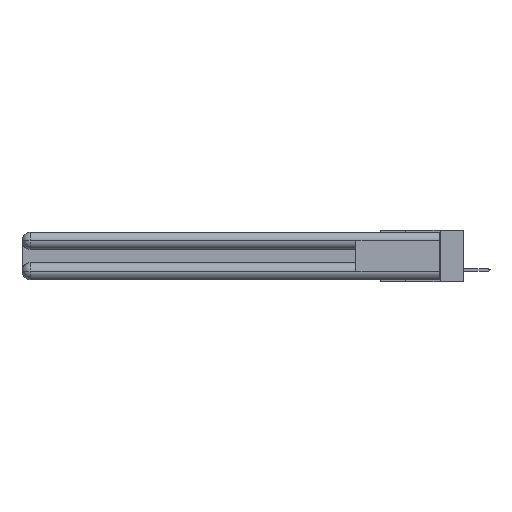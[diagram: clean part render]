
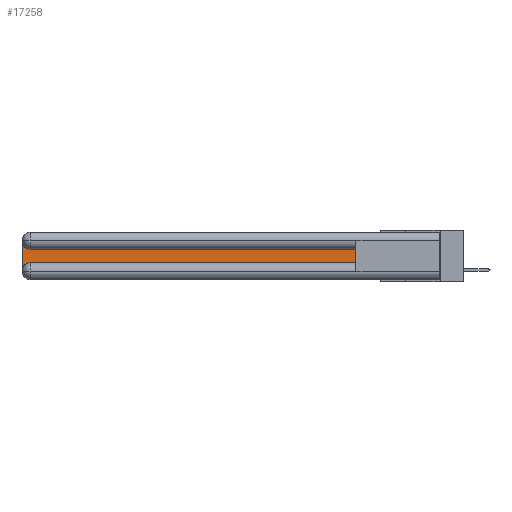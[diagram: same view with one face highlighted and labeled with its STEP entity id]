
A CAD part, left-side view. The second image highlights one B-rep face of the part: STEP entity #17258.
In plain terms, the highlighted planar face has unit normal (-1, 0, 0).
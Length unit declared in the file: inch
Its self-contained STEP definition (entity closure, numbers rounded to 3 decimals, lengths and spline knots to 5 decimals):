
#120 = DIRECTION ( 'NONE',  ( 0., 1., 0. ) ) ;
#713 = ORIENTED_EDGE ( 'NONE', *, *, #8002, .T. ) ;
#2307 = VECTOR ( 'NONE', #11723, 39.37008 ) ;
#2457 = PLANE ( 'NONE',  #19651 ) ;
#3687 = CARTESIAN_POINT ( 'NONE',  ( 0.075, 3., -0.2775 ) ) ;
#3909 = ORIENTED_EDGE ( 'NONE', *, *, #23828, .T. ) ;
#4156 = VERTEX_POINT ( 'NONE', #4724 ) ;
#4724 = CARTESIAN_POINT ( 'NONE',  ( 0.075, 3., -0.0625 ) ) ;
#6380 = LINE ( 'NONE', #19947, #2307 ) ;
#6751 = CARTESIAN_POINT ( 'NONE',  ( 0.075, 0.6, -0.1225 ) ) ;
#7042 = CARTESIAN_POINT ( 'NONE',  ( 0.075, 0.6, -0.2175 ) ) ;
#7141 = VECTOR ( 'NONE', #120, 39.37008 ) ;
#8002 = EDGE_CURVE ( 'NONE', #8964, #11441, #6380, .T. ) ;
#8964 = VERTEX_POINT ( 'NONE', #19576 ) ;
#9056 = DIRECTION ( 'NONE',  ( 0., 0., -1. ) ) ;
#9434 = LINE ( 'NONE', #7042, #18223 ) ;
#9610 = VECTOR ( 'NONE', #18591, 39.37008 ) ;
#9648 = ORIENTED_EDGE ( 'NONE', *, *, #23434, .T. ) ;
#10524 = CIRCLE ( 'NONE', #25186, 0.06 ) ;
#11144 = CIRCLE ( 'NONE', #14987, 0.06 ) ;
#11259 = VERTEX_POINT ( 'NONE', #6751 ) ;
#11441 = VERTEX_POINT ( 'NONE', #24611 ) ;
#11643 = ORIENTED_EDGE ( 'NONE', *, *, #21278, .T. ) ;
#11723 = DIRECTION ( 'NONE',  ( 0., -1., 0. ) ) ;
#12004 = FACE_OUTER_BOUND ( 'NONE', #18512, .T. ) ;
#12564 = DIRECTION ( 'NONE',  ( 1., 0., 0. ) ) ;
#13009 = DIRECTION ( 'NONE',  ( 0., 0., -1. ) ) ;
#13607 = EDGE_CURVE ( 'NONE', #11259, #17030, #15589, .T. ) ;
#14104 = EDGE_CURVE ( 'NONE', #22922, #8964, #10524, .T. ) ;
#14987 = AXIS2_PLACEMENT_3D ( 'NONE', #25508, #12564, #9056 ) ;
#15589 = LINE ( 'NONE', #23904, #7141 ) ;
#16572 = CARTESIAN_POINT ( 'NONE',  ( 0.075, 3., -0.2175 ) ) ;
#16721 = DIRECTION ( 'NONE',  ( 0., 0., 1. ) ) ;
#17030 = VERTEX_POINT ( 'NONE', #26744 ) ;
#17152 = DIRECTION ( 'NONE',  ( 1., 0., 0. ) ) ;
#17258 = ADVANCED_FACE ( 'NONE', ( #12004 ), #2457, .F. ) ;
#18223 = VECTOR ( 'NONE', #16721, 39.37008 ) ;
#18512 = EDGE_LOOP ( 'NONE', ( #26323, #9648, #11643, #19931, #713, #3909 ) ) ;
#18591 = DIRECTION ( 'NONE',  ( 0., 0., -1. ) ) ;
#18625 = DIRECTION ( 'NONE',  ( 0., 0., -1. ) ) ;
#19576 = CARTESIAN_POINT ( 'NONE',  ( 0.075, 2.94, -0.2175 ) ) ;
#19651 = AXIS2_PLACEMENT_3D ( 'NONE', #23027, #26924, #18625 ) ;
#19931 = ORIENTED_EDGE ( 'NONE', *, *, #14104, .T. ) ;
#19947 = CARTESIAN_POINT ( 'NONE',  ( 0.075, 0.6, -0.2175 ) ) ;
#21278 = EDGE_CURVE ( 'NONE', #4156, #22922, #23797, .T. ) ;
#22922 = VERTEX_POINT ( 'NONE', #3687 ) ;
#23027 = CARTESIAN_POINT ( 'NONE',  ( 0.075, 3., -0.1225 ) ) ;
#23434 = EDGE_CURVE ( 'NONE', #17030, #4156, #11144, .T. ) ;
#23797 = LINE ( 'NONE', #16572, #9610 ) ;
#23828 = EDGE_CURVE ( 'NONE', #11441, #11259, #9434, .T. ) ;
#23904 = CARTESIAN_POINT ( 'NONE',  ( 0.075, 0.6, -0.1225 ) ) ;
#24611 = CARTESIAN_POINT ( 'NONE',  ( 0.075, 0.6, -0.2175 ) ) ;
#25186 = AXIS2_PLACEMENT_3D ( 'NONE', #25857, #17152, #13009 ) ;
#25508 = CARTESIAN_POINT ( 'NONE',  ( 0.075, 2.94, -0.0625 ) ) ;
#25857 = CARTESIAN_POINT ( 'NONE',  ( 0.075, 2.94, -0.2775 ) ) ;
#26323 = ORIENTED_EDGE ( 'NONE', *, *, #13607, .T. ) ;
#26744 = CARTESIAN_POINT ( 'NONE',  ( 0.075, 2.94, -0.1225 ) ) ;
#26924 = DIRECTION ( 'NONE',  ( 1., 0., 0. ) ) ;
